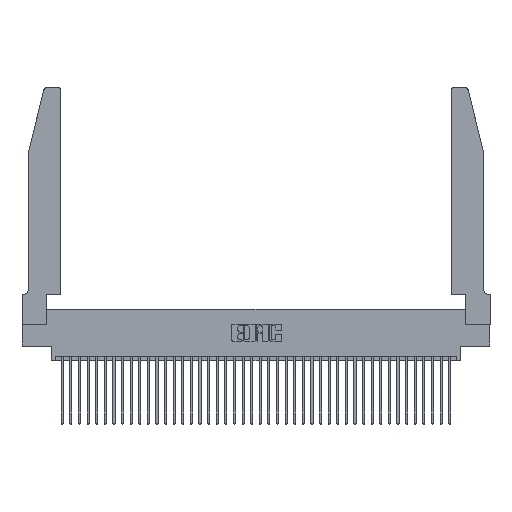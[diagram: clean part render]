
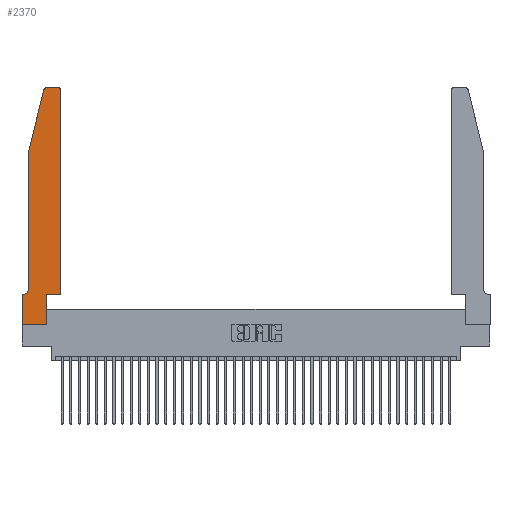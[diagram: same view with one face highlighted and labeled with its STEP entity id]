
A CAD part, top view. The second image highlights one B-rep face of the part: STEP entity #2370.
In plain terms, the highlighted planar face has unit normal (0, 0, 1).
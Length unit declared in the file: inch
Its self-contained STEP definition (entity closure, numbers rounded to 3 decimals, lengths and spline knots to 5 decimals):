
#73 = CIRCLE ( 'NONE', #24083, 0.03 ) ;
#498 = EDGE_CURVE ( 'NONE', #8886, #26673, #19213, .T. ) ;
#520 = DIRECTION ( 'NONE',  ( 0., 0., -1. ) ) ;
#1304 = ORIENTED_EDGE ( 'NONE', *, *, #12290, .T. ) ;
#2321 = DIRECTION ( 'NONE',  ( 1., 0., 0. ) ) ;
#2370 = ADVANCED_FACE ( 'NONE', ( #8696 ), #34438, .T. ) ;
#2730 = DIRECTION ( 'NONE',  ( 0., 0., 1. ) ) ;
#4241 = CARTESIAN_POINT ( 'NONE',  ( 0., 0., 0.37 ) ) ;
#4278 = LINE ( 'NONE', #30092, #6230 ) ;
#4376 = LINE ( 'NONE', #30314, #36727 ) ;
#5008 = VECTOR ( 'NONE', #24154, 39.37008 ) ;
#5746 = CARTESIAN_POINT ( 'NONE',  ( 0., 0.35, 0.37 ) ) ;
#6230 = VECTOR ( 'NONE', #10766, 39.37008 ) ;
#6311 = EDGE_CURVE ( 'NONE', #36554, #8886, #23044, .T. ) ;
#7536 = CARTESIAN_POINT ( 'NONE',  ( 0.0055, 0.42, 0.37 ) ) ;
#7692 = EDGE_CURVE ( 'NONE', #34247, #30864, #32709, .T. ) ;
#7950 = LINE ( 'NONE', #22614, #21727 ) ;
#7972 = EDGE_CURVE ( 'NONE', #37494, #8595, #34170, .T. ) ;
#8595 = VERTEX_POINT ( 'NONE', #16803 ) ;
#8696 = FACE_OUTER_BOUND ( 'NONE', #12994, .T. ) ;
#8738 = CARTESIAN_POINT ( 'NONE',  ( 0.284, 2.72, 0.37 ) ) ;
#8886 = VERTEX_POINT ( 'NONE', #35426 ) ;
#9337 = CARTESIAN_POINT ( 'NONE',  ( 0.4205, 2.72, 0.37 ) ) ;
#9471 = VERTEX_POINT ( 'NONE', #9676 ) ;
#9676 = CARTESIAN_POINT ( 'NONE',  ( 0.284, 2.75, 0.37 ) ) ;
#10366 = EDGE_CURVE ( 'NONE', #29136, #34247, #14816, .T. ) ;
#10424 = CIRCLE ( 'NONE', #20949, 0.03 ) ;
#10766 = DIRECTION ( 'NONE',  ( -1., 0., 0. ) ) ;
#10859 = CARTESIAN_POINT ( 'NONE',  ( 0.2865, 0., 0.37 ) ) ;
#11745 = ORIENTED_EDGE ( 'NONE', *, *, #26304, .T. ) ;
#12238 = DIRECTION ( 'NONE',  ( 0., -1., 0. ) ) ;
#12290 = EDGE_CURVE ( 'NONE', #8595, #28554, #4376, .T. ) ;
#12840 = DIRECTION ( 'NONE',  ( -1., 0., 0. ) ) ;
#12994 = EDGE_LOOP ( 'NONE', ( #24738, #11745, #37521, #31847, #24474, #17372, #19734, #17447, #21782, #1304, #17537, #27910 ) ) ;
#13136 = VECTOR ( 'NONE', #13182, 39.37008 ) ;
#13182 = DIRECTION ( 'NONE',  ( 0., 1., 0. ) ) ;
#13516 = CIRCLE ( 'NONE', #27964, 0.07 ) ;
#14162 = EDGE_CURVE ( 'NONE', #22738, #9471, #4278, .T. ) ;
#14358 = EDGE_CURVE ( 'NONE', #26673, #37494, #35080, .T. ) ;
#14816 = LINE ( 'NONE', #30199, #39727 ) ;
#14826 = CARTESIAN_POINT ( 'NONE',  ( 0., 0., 0.37 ) ) ;
#15884 = AXIS2_PLACEMENT_3D ( 'NONE', #5746, #2730, #22012 ) ;
#16344 = VERTEX_POINT ( 'NONE', #39401 ) ;
#16368 = EDGE_CURVE ( 'NONE', #16344, #22738, #10424, .T. ) ;
#16453 = DIRECTION ( 'NONE',  ( -1., 0., 0. ) ) ;
#16803 = CARTESIAN_POINT ( 'NONE',  ( 0.2865, 0.35, 0.37 ) ) ;
#17372 = ORIENTED_EDGE ( 'NONE', *, *, #6311, .T. ) ;
#17447 = ORIENTED_EDGE ( 'NONE', *, *, #14358, .T. ) ;
#17537 = ORIENTED_EDGE ( 'NONE', *, *, #38004, .T. ) ;
#19213 = LINE ( 'NONE', #14826, #5008 ) ;
#19734 = ORIENTED_EDGE ( 'NONE', *, *, #498, .T. ) ;
#19780 = CARTESIAN_POINT ( 'NONE',  ( 0.2865, 0.35, 0.37 ) ) ;
#20949 = AXIS2_PLACEMENT_3D ( 'NONE', #9337, #31251, #34380 ) ;
#21266 = EDGE_CURVE ( 'NONE', #30864, #36554, #13516, .T. ) ;
#21727 = VECTOR ( 'NONE', #35330, 39.37008 ) ;
#21782 = ORIENTED_EDGE ( 'NONE', *, *, #7972, .T. ) ;
#22012 = DIRECTION ( 'NONE',  ( 1., 0., 0. ) ) ;
#22298 = CARTESIAN_POINT ( 'NONE',  ( 0.4505, 0.35, 0.37 ) ) ;
#22459 = CARTESIAN_POINT ( 'NONE',  ( 0.25487, 2.72718, 0.37 ) ) ;
#22614 = CARTESIAN_POINT ( 'NONE',  ( 0.4505, 0.35, 0.37 ) ) ;
#22738 = VERTEX_POINT ( 'NONE', #31580 ) ;
#23044 = LINE ( 'NONE', #24502, #33322 ) ;
#24083 = AXIS2_PLACEMENT_3D ( 'NONE', #8738, #24088, #2321 ) ;
#24088 = DIRECTION ( 'NONE',  ( 0., 0., 1. ) ) ;
#24154 = DIRECTION ( 'NONE',  ( 0., -1., 0. ) ) ;
#24172 = DIRECTION ( 'NONE',  ( 1., 0., 0. ) ) ;
#24474 = ORIENTED_EDGE ( 'NONE', *, *, #21266, .T. ) ;
#24502 = CARTESIAN_POINT ( 'NONE',  ( 0.0755, 0.35, 0.37 ) ) ;
#24738 = ORIENTED_EDGE ( 'NONE', *, *, #14162, .T. ) ;
#25884 = DIRECTION ( 'NONE',  ( 1., 0., 0. ) ) ;
#26304 = EDGE_CURVE ( 'NONE', #9471, #29136, #73, .T. ) ;
#26673 = VERTEX_POINT ( 'NONE', #34707 ) ;
#27910 = ORIENTED_EDGE ( 'NONE', *, *, #16368, .T. ) ;
#27964 = AXIS2_PLACEMENT_3D ( 'NONE', #7536, #520, #12840 ) ;
#28554 = VERTEX_POINT ( 'NONE', #22298 ) ;
#28766 = VECTOR ( 'NONE', #25884, 39.37008 ) ;
#29136 = VERTEX_POINT ( 'NONE', #22459 ) ;
#30092 = CARTESIAN_POINT ( 'NONE',  ( 0.2605, 2.75, 0.37 ) ) ;
#30199 = CARTESIAN_POINT ( 'NONE',  ( 0.0755, 2., 0.37 ) ) ;
#30314 = CARTESIAN_POINT ( 'NONE',  ( 0.4505, 0.35, 0.37 ) ) ;
#30335 = DIRECTION ( 'NONE',  ( -0.239, -0.971, 0. ) ) ;
#30864 = VERTEX_POINT ( 'NONE', #39714 ) ;
#31251 = DIRECTION ( 'NONE',  ( 0., 0., 1. ) ) ;
#31580 = CARTESIAN_POINT ( 'NONE',  ( 0.4205, 2.75, 0.37 ) ) ;
#31847 = ORIENTED_EDGE ( 'NONE', *, *, #7692, .T. ) ;
#32709 = LINE ( 'NONE', #37632, #38511 ) ;
#33322 = VECTOR ( 'NONE', #16453, 39.37008 ) ;
#34116 = CARTESIAN_POINT ( 'NONE',  ( 0.0755, 2., 0.37 ) ) ;
#34170 = LINE ( 'NONE', #19780, #13136 ) ;
#34247 = VERTEX_POINT ( 'NONE', #34116 ) ;
#34380 = DIRECTION ( 'NONE',  ( 1., 0., 0. ) ) ;
#34438 = PLANE ( 'NONE',  #15884 ) ;
#34707 = CARTESIAN_POINT ( 'NONE',  ( 0., 0., 0.37 ) ) ;
#35080 = LINE ( 'NONE', #4241, #28766 ) ;
#35146 = CARTESIAN_POINT ( 'NONE',  ( 0.0055, 0.35, 0.37 ) ) ;
#35330 = DIRECTION ( 'NONE',  ( 0., 1., 0. ) ) ;
#35426 = CARTESIAN_POINT ( 'NONE',  ( 0., 0.35, 0.37 ) ) ;
#36554 = VERTEX_POINT ( 'NONE', #35146 ) ;
#36727 = VECTOR ( 'NONE', #24172, 39.37008 ) ;
#37494 = VERTEX_POINT ( 'NONE', #10859 ) ;
#37521 = ORIENTED_EDGE ( 'NONE', *, *, #10366, .T. ) ;
#37632 = CARTESIAN_POINT ( 'NONE',  ( 0.0755, 2., 0.37 ) ) ;
#38004 = EDGE_CURVE ( 'NONE', #28554, #16344, #7950, .T. ) ;
#38511 = VECTOR ( 'NONE', #12238, 39.37008 ) ;
#39401 = CARTESIAN_POINT ( 'NONE',  ( 0.4505, 2.72, 0.37 ) ) ;
#39714 = CARTESIAN_POINT ( 'NONE',  ( 0.0755, 0.42, 0.37 ) ) ;
#39727 = VECTOR ( 'NONE', #30335, 39.37008 ) ;
